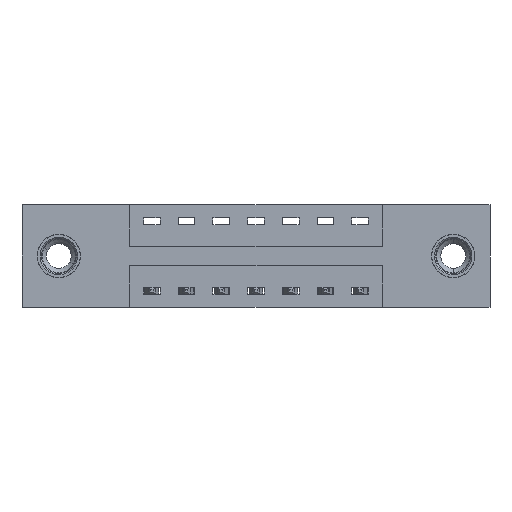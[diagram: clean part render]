
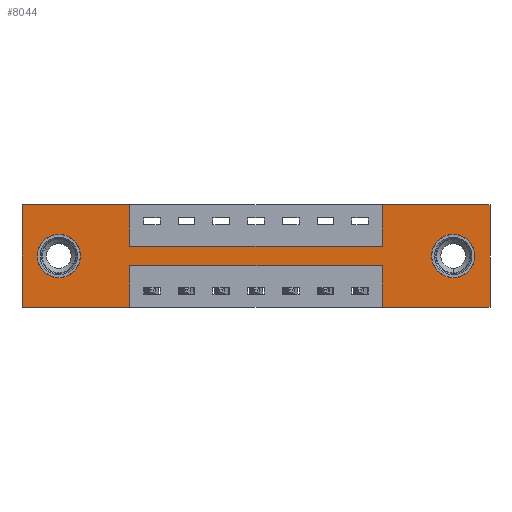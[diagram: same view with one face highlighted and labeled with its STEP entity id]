
A CAD part, front view. The second image highlights one B-rep face of the part: STEP entity #8044.
In plain terms, the highlighted planar face has unit normal (0, -1, 0).
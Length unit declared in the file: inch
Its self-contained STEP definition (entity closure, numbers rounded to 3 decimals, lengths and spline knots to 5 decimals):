
#18 = EDGE_CURVE ( 'NONE', #9595, #4252, #8513, .T. ) ;
#243 = EDGE_CURVE ( 'NONE', #7561, #648, #948, .T. ) ;
#299 = EDGE_CURVE ( 'NONE', #5076, #3466, #1837, .T. ) ;
#504 = VECTOR ( 'NONE', #822, 39.37008 ) ;
#506 = VERTEX_POINT ( 'NONE', #7952 ) ;
#517 = EDGE_CURVE ( 'NONE', #648, #7243, #6819, .T. ) ;
#631 = VECTOR ( 'NONE', #9760, 39.37008 ) ;
#648 = VERTEX_POINT ( 'NONE', #8124 ) ;
#650 = ORIENTED_EDGE ( 'NONE', *, *, #517, .F. ) ;
#705 = CARTESIAN_POINT ( 'NONE',  ( 0., 0., -0.37 ) ) ;
#812 = CIRCLE ( 'NONE', #5464, 0.078 ) ;
#822 = DIRECTION ( 'NONE',  ( 1., 0., 0. ) ) ;
#824 = EDGE_CURVE ( 'NONE', #6987, #506, #8561, .T. ) ;
#872 = FACE_OUTER_BOUND ( 'NONE', #5373, .T. ) ;
#948 = LINE ( 'NONE', #2873, #8640 ) ;
#1104 = CARTESIAN_POINT ( 'NONE',  ( 0.3875, 0., -0.15 ) ) ;
#1209 = LINE ( 'NONE', #6864, #9392 ) ;
#1427 = ORIENTED_EDGE ( 'NONE', *, *, #7663, .F. ) ;
#1489 = DIRECTION ( 'NONE',  ( 0., 1., 0. ) ) ;
#1551 = VECTOR ( 'NONE', #8415, 39.37008 ) ;
#1653 = EDGE_CURVE ( 'NONE', #2840, #8425, #2954, .T. ) ;
#1663 = CIRCLE ( 'NONE', #9401, 0.078 ) ;
#1710 = DIRECTION ( 'NONE',  ( 0., 0., -1. ) ) ;
#1747 = LINE ( 'NONE', #8707, #7791 ) ;
#1789 = EDGE_CURVE ( 'NONE', #5519, #4461, #1747, .T. ) ;
#1837 = CIRCLE ( 'NONE', #10142, 0.078 ) ;
#2184 = DIRECTION ( 'NONE',  ( 0., 1., 0. ) ) ;
#2514 = EDGE_CURVE ( 'NONE', #4638, #7561, #5301, .T. ) ;
#2666 = DIRECTION ( 'NONE',  ( 1., 0., 0. ) ) ;
#2708 = CARTESIAN_POINT ( 'NONE',  ( 0., 0., -0.37 ) ) ;
#2709 = VECTOR ( 'NONE', #8297, 39.37008 ) ;
#2746 = LINE ( 'NONE', #8965, #631 ) ;
#2840 = VERTEX_POINT ( 'NONE', #6225 ) ;
#2868 = CARTESIAN_POINT ( 'NONE',  ( 0.3875, 0., 0. ) ) ;
#2873 = CARTESIAN_POINT ( 'NONE',  ( 1.2975, 0., 0. ) ) ;
#2941 = LINE ( 'NONE', #9058, #2709 ) ;
#2943 = CARTESIAN_POINT ( 'NONE',  ( 1.2975, 0., -0.37 ) ) ;
#2954 = CIRCLE ( 'NONE', #5981, 0.078 ) ;
#3064 = VERTEX_POINT ( 'NONE', #7251 ) ;
#3419 = EDGE_CURVE ( 'NONE', #8425, #2840, #812, .T. ) ;
#3466 = VERTEX_POINT ( 'NONE', #8334 ) ;
#3556 = DIRECTION ( 'NONE',  ( 0., 1., 0. ) ) ;
#3647 = ORIENTED_EDGE ( 'NONE', *, *, #3419, .T. ) ;
#3648 = LINE ( 'NONE', #2868, #1551 ) ;
#3819 = CARTESIAN_POINT ( 'NONE',  ( 0.1325, 0., -0.185 ) ) ;
#3991 = ORIENTED_EDGE ( 'NONE', *, *, #1653, .T. ) ;
#4012 = ORIENTED_EDGE ( 'NONE', *, *, #9333, .F. ) ;
#4074 = CARTESIAN_POINT ( 'NONE',  ( 1.685, 0., 0. ) ) ;
#4114 = CARTESIAN_POINT ( 'NONE',  ( 1.2975, 0., -0.15 ) ) ;
#4165 = ORIENTED_EDGE ( 'NONE', *, *, #9479, .F. ) ;
#4180 = EDGE_CURVE ( 'NONE', #7166, #6987, #8617, .T. ) ;
#4252 = VERTEX_POINT ( 'NONE', #2943 ) ;
#4344 = CARTESIAN_POINT ( 'NONE',  ( 0.1325, 0., -0.263 ) ) ;
#4382 = LINE ( 'NONE', #4074, #8845 ) ;
#4388 = CARTESIAN_POINT ( 'NONE',  ( 0., 0., -0.37 ) ) ;
#4461 = VERTEX_POINT ( 'NONE', #6413 ) ;
#4469 = DIRECTION ( 'NONE',  ( 0., 0., 1. ) ) ;
#4616 = DIRECTION ( 'NONE',  ( 0., 0., 1. ) ) ;
#4628 = DIRECTION ( 'NONE',  ( 0., -1., 0. ) ) ;
#4638 = VERTEX_POINT ( 'NONE', #1104 ) ;
#4731 = CARTESIAN_POINT ( 'NONE',  ( 1.2975, 0., -0.22 ) ) ;
#4740 = EDGE_LOOP ( 'NONE', ( #8923, #7953 ) ) ;
#4767 = EDGE_CURVE ( 'NONE', #506, #4638, #3648, .T. ) ;
#4833 = FACE_BOUND ( 'NONE', #10212, .T. ) ;
#4958 = ORIENTED_EDGE ( 'NONE', *, *, #18, .F. ) ;
#5055 = VECTOR ( 'NONE', #2666, 39.37008 ) ;
#5076 = VERTEX_POINT ( 'NONE', #7948 ) ;
#5138 = EDGE_CURVE ( 'NONE', #7243, #9595, #4382, .T. ) ;
#5219 = ORIENTED_EDGE ( 'NONE', *, *, #5138, .F. ) ;
#5273 = CARTESIAN_POINT ( 'NONE',  ( 0., 0., 0. ) ) ;
#5299 = CARTESIAN_POINT ( 'NONE',  ( 1.685, 0., 0. ) ) ;
#5301 = LINE ( 'NONE', #8201, #5055 ) ;
#5373 = EDGE_LOOP ( 'NONE', ( #1427, #7971, #4012, #4958, #5219, #650, #8591, #5758, #9349, #9853, #6143, #4165 ) ) ;
#5415 = CARTESIAN_POINT ( 'NONE',  ( 1.685, 0., -0.37 ) ) ;
#5439 = EDGE_CURVE ( 'NONE', #3466, #5076, #1663, .T. ) ;
#5464 = AXIS2_PLACEMENT_3D ( 'NONE', #8301, #3556, #9094 ) ;
#5519 = VERTEX_POINT ( 'NONE', #4731 ) ;
#5610 = CARTESIAN_POINT ( 'NONE',  ( 0., 0., 0. ) ) ;
#5758 = ORIENTED_EDGE ( 'NONE', *, *, #2514, .F. ) ;
#5839 = FACE_BOUND ( 'NONE', #4740, .T. ) ;
#5953 = VECTOR ( 'NONE', #9131, 39.37008 ) ;
#5981 = AXIS2_PLACEMENT_3D ( 'NONE', #3819, #9363, #4616 ) ;
#6143 = ORIENTED_EDGE ( 'NONE', *, *, #4180, .F. ) ;
#6224 = CARTESIAN_POINT ( 'NONE',  ( 1.5525, 0., -0.185 ) ) ;
#6225 = CARTESIAN_POINT ( 'NONE',  ( 0.1325, 0., -0.107 ) ) ;
#6408 = VECTOR ( 'NONE', #8089, 39.37008 ) ;
#6413 = CARTESIAN_POINT ( 'NONE',  ( 0.3875, 0., -0.22 ) ) ;
#6819 = LINE ( 'NONE', #5610, #504 ) ;
#6864 = CARTESIAN_POINT ( 'NONE',  ( 0., 0., -0.37 ) ) ;
#6915 = CARTESIAN_POINT ( 'NONE',  ( 1.5525, 0., -0.185 ) ) ;
#6987 = VERTEX_POINT ( 'NONE', #7193 ) ;
#7008 = DIRECTION ( 'NONE',  ( 0., 0., -1. ) ) ;
#7039 = PLANE ( 'NONE',  #7080 ) ;
#7080 = AXIS2_PLACEMENT_3D ( 'NONE', #705, #4628, #7842 ) ;
#7166 = VERTEX_POINT ( 'NONE', #2708 ) ;
#7193 = CARTESIAN_POINT ( 'NONE',  ( 0., 0., 0. ) ) ;
#7243 = VERTEX_POINT ( 'NONE', #5299 ) ;
#7251 = CARTESIAN_POINT ( 'NONE',  ( 0.3875, 0., -0.37 ) ) ;
#7561 = VERTEX_POINT ( 'NONE', #4114 ) ;
#7663 = EDGE_CURVE ( 'NONE', #4461, #3064, #2746, .T. ) ;
#7717 = DIRECTION ( 'NONE',  ( 0., 0., -1. ) ) ;
#7791 = VECTOR ( 'NONE', #8743, 39.37008 ) ;
#7842 = DIRECTION ( 'NONE',  ( 0., 0., -1. ) ) ;
#7948 = CARTESIAN_POINT ( 'NONE',  ( 1.5525, 0., -0.263 ) ) ;
#7952 = CARTESIAN_POINT ( 'NONE',  ( 0.3875, 0., 0. ) ) ;
#7953 = ORIENTED_EDGE ( 'NONE', *, *, #299, .T. ) ;
#7971 = ORIENTED_EDGE ( 'NONE', *, *, #1789, .F. ) ;
#8044 = ADVANCED_FACE ( 'NONE', ( #5839, #4833, #872 ), #7039, .T. ) ;
#8089 = DIRECTION ( 'NONE',  ( -1., 0., 0. ) ) ;
#8124 = CARTESIAN_POINT ( 'NONE',  ( 1.2975, 0., 0. ) ) ;
#8201 = CARTESIAN_POINT ( 'NONE',  ( 0.3875, 0., -0.15 ) ) ;
#8297 = DIRECTION ( 'NONE',  ( 0., 0., 1. ) ) ;
#8301 = CARTESIAN_POINT ( 'NONE',  ( 0.1325, 0., -0.185 ) ) ;
#8304 = CARTESIAN_POINT ( 'NONE',  ( 0., 0., 0. ) ) ;
#8334 = CARTESIAN_POINT ( 'NONE',  ( 1.5525, 0., -0.107 ) ) ;
#8360 = VECTOR ( 'NONE', #9224, 39.37008 ) ;
#8415 = DIRECTION ( 'NONE',  ( 0., 0., -1. ) ) ;
#8425 = VERTEX_POINT ( 'NONE', #4344 ) ;
#8513 = LINE ( 'NONE', #4388, #6408 ) ;
#8561 = LINE ( 'NONE', #8304, #5953 ) ;
#8591 = ORIENTED_EDGE ( 'NONE', *, *, #243, .F. ) ;
#8617 = LINE ( 'NONE', #5273, #8360 ) ;
#8640 = VECTOR ( 'NONE', #4469, 39.37008 ) ;
#8707 = CARTESIAN_POINT ( 'NONE',  ( 0.3875, 0., -0.22 ) ) ;
#8743 = DIRECTION ( 'NONE',  ( -1., 0., 0. ) ) ;
#8845 = VECTOR ( 'NONE', #1710, 39.37008 ) ;
#8923 = ORIENTED_EDGE ( 'NONE', *, *, #5439, .T. ) ;
#8965 = CARTESIAN_POINT ( 'NONE',  ( 0.3875, 0., -0.37 ) ) ;
#9058 = CARTESIAN_POINT ( 'NONE',  ( 1.2975, 0., -0.37 ) ) ;
#9094 = DIRECTION ( 'NONE',  ( 0., 0., 1. ) ) ;
#9131 = DIRECTION ( 'NONE',  ( 1., 0., 0. ) ) ;
#9224 = DIRECTION ( 'NONE',  ( 0., 0., 1. ) ) ;
#9266 = DIRECTION ( 'NONE',  ( -1., 0., 0. ) ) ;
#9333 = EDGE_CURVE ( 'NONE', #4252, #5519, #2941, .T. ) ;
#9349 = ORIENTED_EDGE ( 'NONE', *, *, #4767, .F. ) ;
#9363 = DIRECTION ( 'NONE',  ( 0., 1., 0. ) ) ;
#9392 = VECTOR ( 'NONE', #9266, 39.37008 ) ;
#9401 = AXIS2_PLACEMENT_3D ( 'NONE', #6224, #1489, #7008 ) ;
#9479 = EDGE_CURVE ( 'NONE', #3064, #7166, #1209, .T. ) ;
#9595 = VERTEX_POINT ( 'NONE', #5415 ) ;
#9760 = DIRECTION ( 'NONE',  ( 0., 0., -1. ) ) ;
#9853 = ORIENTED_EDGE ( 'NONE', *, *, #824, .F. ) ;
#10142 = AXIS2_PLACEMENT_3D ( 'NONE', #6915, #2184, #7717 ) ;
#10212 = EDGE_LOOP ( 'NONE', ( #3991, #3647 ) ) ;
